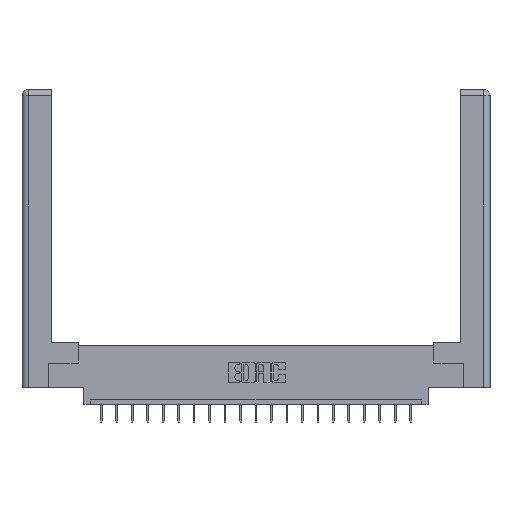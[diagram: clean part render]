
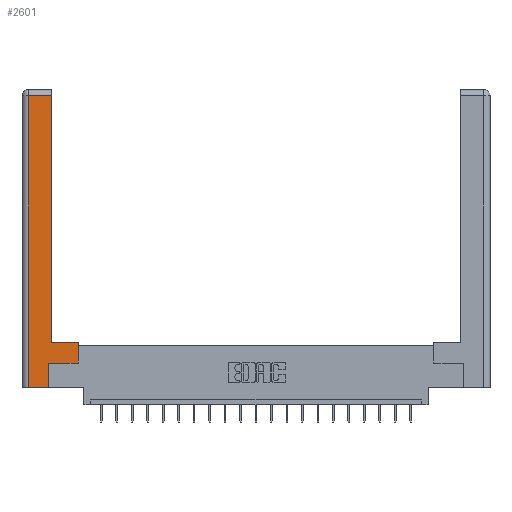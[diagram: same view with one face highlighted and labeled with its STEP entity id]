
A CAD part, top view. The second image highlights one B-rep face of the part: STEP entity #2601.
In plain terms, the highlighted planar face has unit normal (0, 0, 1).
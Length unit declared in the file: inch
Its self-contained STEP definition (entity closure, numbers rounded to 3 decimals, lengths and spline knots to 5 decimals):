
#13 = VECTOR ( 'NONE', #16356, 39.37008 ) ;
#81 = VECTOR ( 'NONE', #8386, 39.37008 ) ;
#400 = VERTEX_POINT ( 'NONE', #15029 ) ;
#621 = EDGE_CURVE ( 'NONE', #17847, #1084, #18038, .T. ) ;
#938 = DIRECTION ( 'NONE',  ( 0., -1., 0. ) ) ;
#1084 = VERTEX_POINT ( 'NONE', #1314 ) ;
#1085 = FACE_OUTER_BOUND ( 'NONE', #6089, .T. ) ;
#1314 = CARTESIAN_POINT ( 'NONE',  ( 0.0615, 2.94, 0. ) ) ;
#1365 = DIRECTION ( 'NONE',  ( -1., 0., 0. ) ) ;
#1375 = EDGE_CURVE ( 'NONE', #400, #2095, #15970, .T. ) ;
#1535 = VERTEX_POINT ( 'NONE', #11855 ) ;
#1907 = ORIENTED_EDGE ( 'NONE', *, *, #14589, .T. ) ;
#2048 = ORIENTED_EDGE ( 'NONE', *, *, #9102, .T. ) ;
#2095 = VERTEX_POINT ( 'NONE', #20129 ) ;
#2484 = LINE ( 'NONE', #10177, #5295 ) ;
#2601 = ADVANCED_FACE ( 'NONE', ( #1085 ), #18824, .F. ) ;
#3749 = VECTOR ( 'NONE', #8040, 39.37008 ) ;
#3803 = DIRECTION ( 'NONE',  ( 1., 0., 0. ) ) ;
#4023 = LINE ( 'NONE', #6787, #7334 ) ;
#4905 = CARTESIAN_POINT ( 'NONE',  ( 0.565, 0.45, 0. ) ) ;
#5233 = CARTESIAN_POINT ( 'NONE',  ( 0.295, 3., 0. ) ) ;
#5274 = VERTEX_POINT ( 'NONE', #18369 ) ;
#5295 = VECTOR ( 'NONE', #13466, 39.37008 ) ;
#5633 = LINE ( 'NONE', #4905, #13 ) ;
#5989 = CARTESIAN_POINT ( 'NONE',  ( 0.295, 0.45, 0. ) ) ;
#6089 = EDGE_LOOP ( 'NONE', ( #17067, #9231, #17721, #1907, #9822, #9451, #2048, #7873 ) ) ;
#6230 = CARTESIAN_POINT ( 'NONE',  ( 0.295, 2.94, 0. ) ) ;
#6787 = CARTESIAN_POINT ( 'NONE',  ( 0.565, 0.245, 0. ) ) ;
#7334 = VECTOR ( 'NONE', #3803, 39.37008 ) ;
#7453 = CARTESIAN_POINT ( 'NONE',  ( 0.265, 0., 0. ) ) ;
#7774 = VECTOR ( 'NONE', #12737, 39.37008 ) ;
#7873 = ORIENTED_EDGE ( 'NONE', *, *, #1375, .T. ) ;
#8040 = DIRECTION ( 'NONE',  ( -1., 0., 0. ) ) ;
#8386 = DIRECTION ( 'NONE',  ( 0., 1., 0. ) ) ;
#9006 = CARTESIAN_POINT ( 'NONE',  ( 0.0615, 0., 0. ) ) ;
#9102 = EDGE_CURVE ( 'NONE', #5274, #400, #5633, .T. ) ;
#9231 = ORIENTED_EDGE ( 'NONE', *, *, #621, .T. ) ;
#9451 = ORIENTED_EDGE ( 'NONE', *, *, #14538, .T. ) ;
#9822 = ORIENTED_EDGE ( 'NONE', *, *, #13363, .T. ) ;
#10177 = CARTESIAN_POINT ( 'NONE',  ( 0.265, 0., 0. ) ) ;
#11044 = VECTOR ( 'NONE', #19599, 39.37008 ) ;
#11568 = LINE ( 'NONE', #11616, #11044 ) ;
#11616 = CARTESIAN_POINT ( 'NONE',  ( 0.265, 0.245, 0. ) ) ;
#11855 = CARTESIAN_POINT ( 'NONE',  ( 0.265, 0.245, 0. ) ) ;
#12594 = LINE ( 'NONE', #5233, #81 ) ;
#12631 = AXIS2_PLACEMENT_3D ( 'NONE', #16140, #19477, #1365 ) ;
#12737 = DIRECTION ( 'NONE',  ( -1., 0., 0. ) ) ;
#13363 = EDGE_CURVE ( 'NONE', #20389, #1535, #11568, .T. ) ;
#13466 = DIRECTION ( 'NONE',  ( 1., 0., 0. ) ) ;
#14538 = EDGE_CURVE ( 'NONE', #1535, #5274, #4023, .T. ) ;
#14589 = EDGE_CURVE ( 'NONE', #18305, #20389, #2484, .T. ) ;
#15029 = CARTESIAN_POINT ( 'NONE',  ( 0.565, 0.45, 0. ) ) ;
#15410 = EDGE_CURVE ( 'NONE', #1084, #18305, #17506, .T. ) ;
#15970 = LINE ( 'NONE', #5989, #7774 ) ;
#16140 = CARTESIAN_POINT ( 'NONE',  ( 0., 0., 0. ) ) ;
#16356 = DIRECTION ( 'NONE',  ( 0., 1., 0. ) ) ;
#17067 = ORIENTED_EDGE ( 'NONE', *, *, #17190, .T. ) ;
#17190 = EDGE_CURVE ( 'NONE', #2095, #17847, #12594, .T. ) ;
#17506 = LINE ( 'NONE', #9006, #20574 ) ;
#17721 = ORIENTED_EDGE ( 'NONE', *, *, #15410, .T. ) ;
#17732 = CARTESIAN_POINT ( 'NONE',  ( 0.0615, 0., 0. ) ) ;
#17847 = VERTEX_POINT ( 'NONE', #6230 ) ;
#18038 = LINE ( 'NONE', #18370, #3749 ) ;
#18305 = VERTEX_POINT ( 'NONE', #17732 ) ;
#18369 = CARTESIAN_POINT ( 'NONE',  ( 0.565, 0.245, 0. ) ) ;
#18370 = CARTESIAN_POINT ( 'NONE',  ( 0.0615, 2.94, 0. ) ) ;
#18824 = PLANE ( 'NONE',  #12631 ) ;
#19477 = DIRECTION ( 'NONE',  ( 0., 0., -1. ) ) ;
#19599 = DIRECTION ( 'NONE',  ( 0., 1., 0. ) ) ;
#20129 = CARTESIAN_POINT ( 'NONE',  ( 0.295, 0.45, 0. ) ) ;
#20389 = VERTEX_POINT ( 'NONE', #7453 ) ;
#20574 = VECTOR ( 'NONE', #938, 39.37008 ) ;
